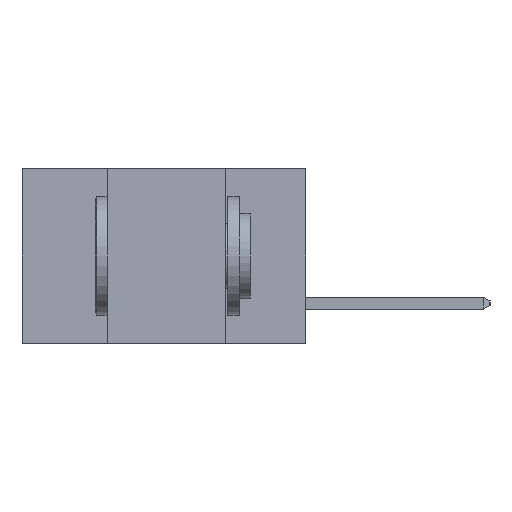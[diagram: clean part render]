
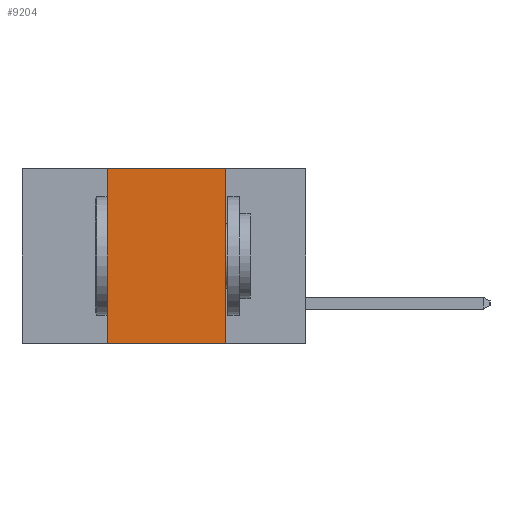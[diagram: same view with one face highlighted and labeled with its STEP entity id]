
A CAD part, left-side view. The second image highlights one B-rep face of the part: STEP entity #9204.
In plain terms, the highlighted planar face has unit normal (-1, 0, 0).
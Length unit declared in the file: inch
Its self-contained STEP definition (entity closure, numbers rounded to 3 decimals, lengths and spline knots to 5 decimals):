
#950 = CARTESIAN_POINT ( 'NONE',  ( 0., 0.42, 0. ) ) ;
#1090 = VECTOR ( 'NONE', #8674, 39.37008 ) ;
#1288 = CARTESIAN_POINT ( 'NONE',  ( 0., 0.42, -0.37 ) ) ;
#1499 = EDGE_CURVE ( 'NONE', #5753, #5181, #10018, .T. ) ;
#1888 = EDGE_CURVE ( 'NONE', #5287, #2480, #2160, .T. ) ;
#2160 = LINE ( 'NONE', #4460, #10257 ) ;
#2480 = VERTEX_POINT ( 'NONE', #3765 ) ;
#2603 = CARTESIAN_POINT ( 'NONE',  ( 0., 0.17, 0. ) ) ;
#2971 = DIRECTION ( 'NONE',  ( 0., -1., 0. ) ) ;
#3057 = DIRECTION ( 'NONE',  ( 0., -1., 0. ) ) ;
#3131 = VECTOR ( 'NONE', #2971, 39.37008 ) ;
#3372 = CARTESIAN_POINT ( 'NONE',  ( 0., 0.6, 0. ) ) ;
#3765 = CARTESIAN_POINT ( 'NONE',  ( 0., 0.17, -0.37 ) ) ;
#3956 = DIRECTION ( 'NONE',  ( 0., 0., -1. ) ) ;
#4146 = CARTESIAN_POINT ( 'NONE',  ( 0., 0.6, -0.37 ) ) ;
#4244 = DIRECTION ( 'NONE',  ( 1., 0., 0. ) ) ;
#4460 = CARTESIAN_POINT ( 'NONE',  ( 0., 0.17, 0. ) ) ;
#4639 = EDGE_CURVE ( 'NONE', #5753, #2480, #8681, .T. ) ;
#5181 = VERTEX_POINT ( 'NONE', #950 ) ;
#5287 = VERTEX_POINT ( 'NONE', #2603 ) ;
#5603 = ORIENTED_EDGE ( 'NONE', *, *, #7040, .F. ) ;
#5621 = ORIENTED_EDGE ( 'NONE', *, *, #1888, .F. ) ;
#5753 = VERTEX_POINT ( 'NONE', #1288 ) ;
#6503 = EDGE_LOOP ( 'NONE', ( #5621, #5603, #8404, #9315 ) ) ;
#7040 = EDGE_CURVE ( 'NONE', #5181, #5287, #9586, .T. ) ;
#8098 = CARTESIAN_POINT ( 'NONE',  ( 0., 0.42, 0. ) ) ;
#8206 = VECTOR ( 'NONE', #3057, 39.37008 ) ;
#8310 = PLANE ( 'NONE',  #10034 ) ;
#8404 = ORIENTED_EDGE ( 'NONE', *, *, #1499, .F. ) ;
#8674 = DIRECTION ( 'NONE',  ( 0., 0., 1. ) ) ;
#8681 = LINE ( 'NONE', #4146, #8206 ) ;
#9196 = FACE_OUTER_BOUND ( 'NONE', #6503, .T. ) ;
#9204 = ADVANCED_FACE ( 'NONE', ( #9196 ), #8310, .F. ) ;
#9315 = ORIENTED_EDGE ( 'NONE', *, *, #4639, .T. ) ;
#9586 = LINE ( 'NONE', #10157, #3131 ) ;
#9811 = DIRECTION ( 'NONE',  ( 0., 0., -1. ) ) ;
#10018 = LINE ( 'NONE', #8098, #1090 ) ;
#10034 = AXIS2_PLACEMENT_3D ( 'NONE', #3372, #4244, #9811 ) ;
#10157 = CARTESIAN_POINT ( 'NONE',  ( 0., 0.6, 0. ) ) ;
#10257 = VECTOR ( 'NONE', #3956, 39.37008 ) ;
